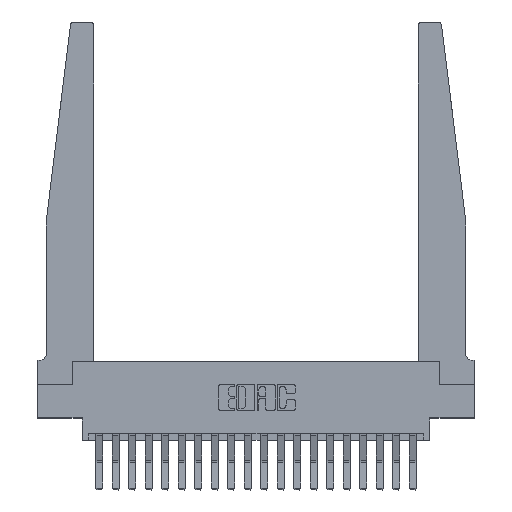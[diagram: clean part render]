
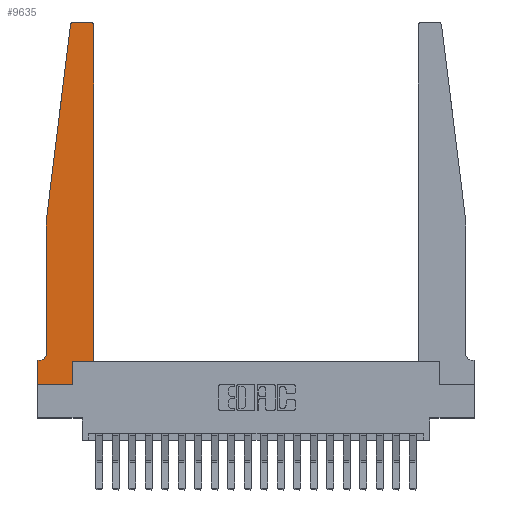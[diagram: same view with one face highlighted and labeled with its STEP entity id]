
A CAD part, top view. The second image highlights one B-rep face of the part: STEP entity #9635.
In plain terms, the highlighted planar face has unit normal (0, 0, 1).
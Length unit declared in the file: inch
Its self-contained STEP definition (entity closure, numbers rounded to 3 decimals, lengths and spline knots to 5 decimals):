
#28 = CARTESIAN_POINT ( 'NONE',  ( 0.27653, 2.72, 0.37 ) ) ;
#142 = LINE ( 'NONE', #472, #17797 ) ;
#472 = CARTESIAN_POINT ( 'NONE',  ( 0.065, 1.25, 0.37 ) ) ;
#524 = CARTESIAN_POINT ( 'NONE',  ( 0.015, 0.2375, 0.37 ) ) ;
#529 = EDGE_CURVE ( 'NONE', #5251, #6361, #9500, .T. ) ;
#892 = CARTESIAN_POINT ( 'NONE',  ( 0.015, 0.1875, 0.37 ) ) ;
#1141 = DIRECTION ( 'NONE',  ( 0., -1., 0. ) ) ;
#1324 = EDGE_CURVE ( 'NONE', #2612, #7269, #3804, .T. ) ;
#1588 = LINE ( 'NONE', #4953, #7938 ) ;
#1841 = CARTESIAN_POINT ( 'NONE',  ( 0.065, 1.25, 0.37 ) ) ;
#2029 = CARTESIAN_POINT ( 'NONE',  ( 0., 0., 0.37 ) ) ;
#2199 = CARTESIAN_POINT ( 'NONE',  ( 0.425, 2.72, 0.37 ) ) ;
#2211 = EDGE_CURVE ( 'NONE', #6113, #2612, #1588, .T. ) ;
#2475 = AXIS2_PLACEMENT_3D ( 'NONE', #28, #8394, #14910 ) ;
#2501 = EDGE_CURVE ( 'NONE', #20032, #5251, #10924, .T. ) ;
#2559 = CARTESIAN_POINT ( 'NONE',  ( 0.065, 1.25, 0.37 ) ) ;
#2612 = VERTEX_POINT ( 'NONE', #3494 ) ;
#2759 = VECTOR ( 'NONE', #1141, 39.37008 ) ;
#2875 = CARTESIAN_POINT ( 'NONE',  ( 0.065, 0.1875, 0.37 ) ) ;
#3494 = CARTESIAN_POINT ( 'NONE',  ( 0.425, 0.18, 0.37 ) ) ;
#3545 = ORIENTED_EDGE ( 'NONE', *, *, #1324, .T. ) ;
#3546 = ORIENTED_EDGE ( 'NONE', *, *, #16427, .T. ) ;
#3740 = VERTEX_POINT ( 'NONE', #2559 ) ;
#3804 = LINE ( 'NONE', #16780, #13480 ) ;
#3828 = CIRCLE ( 'NONE', #16001, 0.03 ) ;
#4083 = EDGE_LOOP ( 'NONE', ( #3546, #4394, #18470, #20042, #6947, #7134, #13702, #11823, #9496, #20921, #3545, #17470 ) ) ;
#4199 = EDGE_CURVE ( 'NONE', #13598, #20032, #11255, .T. ) ;
#4394 = ORIENTED_EDGE ( 'NONE', *, *, #4819, .T. ) ;
#4819 = EDGE_CURVE ( 'NONE', #5182, #11699, #5595, .T. ) ;
#4953 = CARTESIAN_POINT ( 'NONE',  ( 0.425, 0.18, 0.37 ) ) ;
#5182 = VERTEX_POINT ( 'NONE', #6705 ) ;
#5197 = DIRECTION ( 'NONE',  ( -0.122, -0.992, 0. ) ) ;
#5233 = CARTESIAN_POINT ( 'NONE',  ( 0.2605, 0.18, 0.37 ) ) ;
#5251 = VERTEX_POINT ( 'NONE', #2029 ) ;
#5299 = DIRECTION ( 'NONE',  ( 0., 0., -1. ) ) ;
#5415 = CARTESIAN_POINT ( 'NONE',  ( 0.25, 2.75, 0.37 ) ) ;
#5595 = CIRCLE ( 'NONE', #2475, 0.03 ) ;
#5792 = CARTESIAN_POINT ( 'NONE',  ( 0.395, 2.75, 0.37 ) ) ;
#6027 = CARTESIAN_POINT ( 'NONE',  ( 0., 0., 0.37 ) ) ;
#6113 = VERTEX_POINT ( 'NONE', #15687 ) ;
#6361 = VERTEX_POINT ( 'NONE', #18137 ) ;
#6403 = CARTESIAN_POINT ( 'NONE',  ( 0.065, 0.2375, 0.37 ) ) ;
#6642 = CARTESIAN_POINT ( 'NONE',  ( 0., 0., 0.37 ) ) ;
#6705 = CARTESIAN_POINT ( 'NONE',  ( 0.27653, 2.75, 0.37 ) ) ;
#6947 = ORIENTED_EDGE ( 'NONE', *, *, #20630, .T. ) ;
#7068 = LINE ( 'NONE', #5415, #7889 ) ;
#7134 = ORIENTED_EDGE ( 'NONE', *, *, #4199, .T. ) ;
#7269 = VERTEX_POINT ( 'NONE', #2199 ) ;
#7317 = VECTOR ( 'NONE', #18073, 39.37008 ) ;
#7889 = VECTOR ( 'NONE', #20307, 39.37008 ) ;
#7938 = VECTOR ( 'NONE', #13441, 39.37008 ) ;
#8017 = VECTOR ( 'NONE', #11883, 39.37008 ) ;
#8394 = DIRECTION ( 'NONE',  ( 0., 0., 1. ) ) ;
#8833 = DIRECTION ( 'NONE',  ( 0., 0., 1. ) ) ;
#9363 = AXIS2_PLACEMENT_3D ( 'NONE', #524, #5299, #20287 ) ;
#9496 = ORIENTED_EDGE ( 'NONE', *, *, #19949, .T. ) ;
#9500 = LINE ( 'NONE', #6027, #20224 ) ;
#9635 = ADVANCED_FACE ( 'NONE', ( #20141 ), #13524, .T. ) ;
#9708 = CIRCLE ( 'NONE', #9363, 0.05 ) ;
#10144 = DIRECTION ( 'NONE',  ( 1., 0., 0. ) ) ;
#10924 = LINE ( 'NONE', #6642, #2759 ) ;
#11255 = LINE ( 'NONE', #2875, #7317 ) ;
#11639 = VERTEX_POINT ( 'NONE', #6403 ) ;
#11659 = CARTESIAN_POINT ( 'NONE',  ( 0., 0.1875, 0.37 ) ) ;
#11699 = VERTEX_POINT ( 'NONE', #18569 ) ;
#11738 = EDGE_CURVE ( 'NONE', #11699, #3740, #17049, .T. ) ;
#11823 = ORIENTED_EDGE ( 'NONE', *, *, #529, .T. ) ;
#11883 = DIRECTION ( 'NONE',  ( 0., 1., 0. ) ) ;
#12041 = VERTEX_POINT ( 'NONE', #5792 ) ;
#12082 = LINE ( 'NONE', #5233, #8017 ) ;
#13382 = DIRECTION ( 'NONE',  ( 0., 1., 0. ) ) ;
#13441 = DIRECTION ( 'NONE',  ( 1., 0., 0. ) ) ;
#13480 = VECTOR ( 'NONE', #13382, 39.37008 ) ;
#13524 = PLANE ( 'NONE',  #16567 ) ;
#13598 = VERTEX_POINT ( 'NONE', #892 ) ;
#13702 = ORIENTED_EDGE ( 'NONE', *, *, #2501, .T. ) ;
#14910 = DIRECTION ( 'NONE',  ( 1., 0., 0. ) ) ;
#14916 = DIRECTION ( 'NONE',  ( 0., 0., 1. ) ) ;
#15141 = DIRECTION ( 'NONE',  ( 1., 0., 0. ) ) ;
#15582 = CARTESIAN_POINT ( 'NONE',  ( 0., 0.1875, 0.37 ) ) ;
#15687 = CARTESIAN_POINT ( 'NONE',  ( 0.2605, 0.18, 0.37 ) ) ;
#16001 = AXIS2_PLACEMENT_3D ( 'NONE', #20330, #14916, #15141 ) ;
#16129 = VECTOR ( 'NONE', #5197, 39.37008 ) ;
#16427 = EDGE_CURVE ( 'NONE', #12041, #5182, #7068, .T. ) ;
#16567 = AXIS2_PLACEMENT_3D ( 'NONE', #15582, #8833, #10144 ) ;
#16780 = CARTESIAN_POINT ( 'NONE',  ( 0.425, 0.18, 0.37 ) ) ;
#17049 = LINE ( 'NONE', #1841, #16129 ) ;
#17166 = EDGE_CURVE ( 'NONE', #3740, #11639, #142, .T. ) ;
#17329 = DIRECTION ( 'NONE',  ( 1., 0., 0. ) ) ;
#17470 = ORIENTED_EDGE ( 'NONE', *, *, #19872, .T. ) ;
#17797 = VECTOR ( 'NONE', #19922, 39.37008 ) ;
#18073 = DIRECTION ( 'NONE',  ( -1., 0., 0. ) ) ;
#18137 = CARTESIAN_POINT ( 'NONE',  ( 0.2605, 0., 0.37 ) ) ;
#18470 = ORIENTED_EDGE ( 'NONE', *, *, #11738, .T. ) ;
#18569 = CARTESIAN_POINT ( 'NONE',  ( 0.24675, 2.72367, 0.37 ) ) ;
#19872 = EDGE_CURVE ( 'NONE', #7269, #12041, #3828, .T. ) ;
#19922 = DIRECTION ( 'NONE',  ( 0., -1., 0. ) ) ;
#19949 = EDGE_CURVE ( 'NONE', #6361, #6113, #12082, .T. ) ;
#20032 = VERTEX_POINT ( 'NONE', #11659 ) ;
#20042 = ORIENTED_EDGE ( 'NONE', *, *, #17166, .T. ) ;
#20141 = FACE_OUTER_BOUND ( 'NONE', #4083, .T. ) ;
#20224 = VECTOR ( 'NONE', #17329, 39.37008 ) ;
#20287 = DIRECTION ( 'NONE',  ( -1., 0., 0. ) ) ;
#20307 = DIRECTION ( 'NONE',  ( -1., 0., 0. ) ) ;
#20330 = CARTESIAN_POINT ( 'NONE',  ( 0.395, 2.72, 0.37 ) ) ;
#20630 = EDGE_CURVE ( 'NONE', #11639, #13598, #9708, .T. ) ;
#20921 = ORIENTED_EDGE ( 'NONE', *, *, #2211, .T. ) ;
